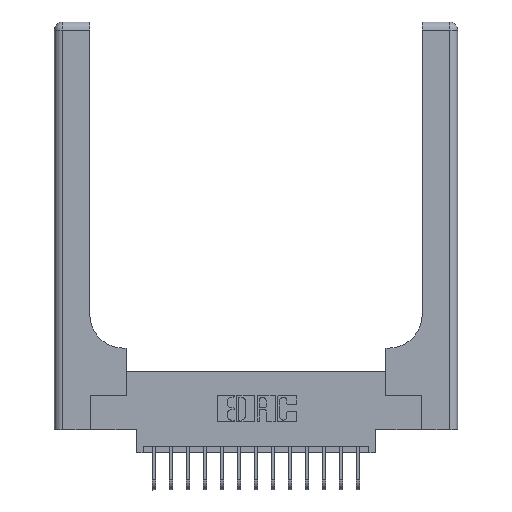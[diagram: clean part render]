
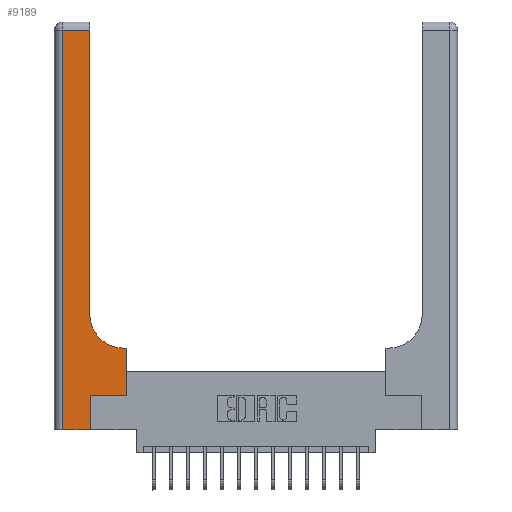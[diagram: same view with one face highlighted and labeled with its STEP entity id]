
A CAD part, top view. The second image highlights one B-rep face of the part: STEP entity #9189.
In plain terms, the highlighted planar face has unit normal (0, 0, 1).
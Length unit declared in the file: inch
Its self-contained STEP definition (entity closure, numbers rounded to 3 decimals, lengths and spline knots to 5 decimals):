
#26 = DIRECTION ( 'NONE',  ( 0., 0., -1. ) ) ;
#106 = CARTESIAN_POINT ( 'NONE',  ( 0.528, 0.25, 0.37 ) ) ;
#921 = VERTEX_POINT ( 'NONE', #11415 ) ;
#1270 = ORIENTED_EDGE ( 'NONE', *, *, #2033, .T. ) ;
#1324 = EDGE_CURVE ( 'NONE', #6707, #921, #7881, .T. ) ;
#1332 = CARTESIAN_POINT ( 'NONE',  ( 0.265, 0.25, 0.37 ) ) ;
#1416 = DIRECTION ( 'NONE',  ( 1., 0., 0. ) ) ;
#1627 = LINE ( 'NONE', #106, #6338 ) ;
#2033 = EDGE_CURVE ( 'NONE', #17599, #7327, #18472, .T. ) ;
#2275 = VERTEX_POINT ( 'NONE', #7486 ) ;
#2289 = EDGE_CURVE ( 'NONE', #13802, #9643, #6070, .T. ) ;
#2573 = VERTEX_POINT ( 'NONE', #11495 ) ;
#2879 = CARTESIAN_POINT ( 'NONE',  ( 0., 3., 0.37 ) ) ;
#3080 = EDGE_CURVE ( 'NONE', #2573, #6707, #17829, .T. ) ;
#3231 = ORIENTED_EDGE ( 'NONE', *, *, #6106, .T. ) ;
#3251 = DIRECTION ( 'NONE',  ( 0., 1., 0. ) ) ;
#3326 = CARTESIAN_POINT ( 'NONE',  ( 0.06, 3., 0.37 ) ) ;
#4124 = CARTESIAN_POINT ( 'NONE',  ( 0.528, 0.25, 0.37 ) ) ;
#4389 = FACE_OUTER_BOUND ( 'NONE', #15207, .T. ) ;
#4398 = EDGE_CURVE ( 'NONE', #5051, #17599, #1627, .T. ) ;
#4751 = DIRECTION ( 'NONE',  ( 0., -1., 0. ) ) ;
#4932 = ORIENTED_EDGE ( 'NONE', *, *, #8261, .T. ) ;
#5051 = VERTEX_POINT ( 'NONE', #4124 ) ;
#5181 = DIRECTION ( 'NONE',  ( 1., 0., 0. ) ) ;
#5896 = ORIENTED_EDGE ( 'NONE', *, *, #12266, .T. ) ;
#6070 = LINE ( 'NONE', #8895, #14020 ) ;
#6106 = EDGE_CURVE ( 'NONE', #7327, #2275, #11852, .T. ) ;
#6338 = VECTOR ( 'NONE', #3251, 39.37008 ) ;
#6693 = CARTESIAN_POINT ( 'NONE',  ( 0.26, 3., 0.37 ) ) ;
#6707 = VERTEX_POINT ( 'NONE', #19014 ) ;
#6904 = DIRECTION ( 'NONE',  ( 0., 1., 0. ) ) ;
#6920 = VECTOR ( 'NONE', #4751, 39.37008 ) ;
#7141 = CARTESIAN_POINT ( 'NONE',  ( 0.26, 0.6, 0.37 ) ) ;
#7327 = VERTEX_POINT ( 'NONE', #10145 ) ;
#7475 = DIRECTION ( 'NONE',  ( 0., 0., -1. ) ) ;
#7486 = CARTESIAN_POINT ( 'NONE',  ( 0.26, 0.85, 0.37 ) ) ;
#7881 = LINE ( 'NONE', #3326, #6920 ) ;
#8017 = EDGE_CURVE ( 'NONE', #921, #13802, #8300, .T. ) ;
#8110 = CARTESIAN_POINT ( 'NONE',  ( 0.528, 0.6, 0.37 ) ) ;
#8261 = EDGE_CURVE ( 'NONE', #9643, #5051, #15157, .T. ) ;
#8300 = LINE ( 'NONE', #18966, #10234 ) ;
#8419 = ORIENTED_EDGE ( 'NONE', *, *, #4398, .T. ) ;
#8660 = VECTOR ( 'NONE', #1416, 39.37008 ) ;
#8895 = CARTESIAN_POINT ( 'NONE',  ( 0.265, 0., 0.37 ) ) ;
#9189 = ADVANCED_FACE ( 'NONE', ( #4389 ), #16714, .F. ) ;
#9643 = VERTEX_POINT ( 'NONE', #15859 ) ;
#10145 = CARTESIAN_POINT ( 'NONE',  ( 0.51, 0.6, 0.37 ) ) ;
#10156 = CARTESIAN_POINT ( 'NONE',  ( 0., 2.94, 0.37 ) ) ;
#10234 = VECTOR ( 'NONE', #5181, 39.37008 ) ;
#10380 = ORIENTED_EDGE ( 'NONE', *, *, #3080, .T. ) ;
#10494 = VECTOR ( 'NONE', #19528, 39.37008 ) ;
#10781 = VECTOR ( 'NONE', #18287, 39.37008 ) ;
#11415 = CARTESIAN_POINT ( 'NONE',  ( 0.06, 0., 0.37 ) ) ;
#11495 = CARTESIAN_POINT ( 'NONE',  ( 0.26, 2.94, 0.37 ) ) ;
#11852 = CIRCLE ( 'NONE', #13165, 0.25 ) ;
#12220 = AXIS2_PLACEMENT_3D ( 'NONE', #2879, #26, #15277 ) ;
#12266 = EDGE_CURVE ( 'NONE', #2275, #2573, #14577, .T. ) ;
#12301 = CARTESIAN_POINT ( 'NONE',  ( 0.51, 0.85, 0.37 ) ) ;
#13165 = AXIS2_PLACEMENT_3D ( 'NONE', #12301, #7475, #17061 ) ;
#13802 = VERTEX_POINT ( 'NONE', #16172 ) ;
#14020 = VECTOR ( 'NONE', #15351, 39.37008 ) ;
#14113 = ORIENTED_EDGE ( 'NONE', *, *, #8017, .T. ) ;
#14577 = LINE ( 'NONE', #6693, #15533 ) ;
#15157 = LINE ( 'NONE', #1332, #8660 ) ;
#15207 = EDGE_LOOP ( 'NONE', ( #5896, #10380, #17522, #14113, #15241, #4932, #8419, #1270, #3231 ) ) ;
#15241 = ORIENTED_EDGE ( 'NONE', *, *, #2289, .T. ) ;
#15277 = DIRECTION ( 'NONE',  ( -1., 0., 0. ) ) ;
#15351 = DIRECTION ( 'NONE',  ( 0., 1., 0. ) ) ;
#15533 = VECTOR ( 'NONE', #6904, 39.37008 ) ;
#15859 = CARTESIAN_POINT ( 'NONE',  ( 0.265, 0.25, 0.37 ) ) ;
#16172 = CARTESIAN_POINT ( 'NONE',  ( 0.265, 0., 0.37 ) ) ;
#16714 = PLANE ( 'NONE',  #12220 ) ;
#17061 = DIRECTION ( 'NONE',  ( 1., 0., 0. ) ) ;
#17522 = ORIENTED_EDGE ( 'NONE', *, *, #1324, .T. ) ;
#17599 = VERTEX_POINT ( 'NONE', #8110 ) ;
#17829 = LINE ( 'NONE', #10156, #10494 ) ;
#18287 = DIRECTION ( 'NONE',  ( -1., 0., 0. ) ) ;
#18472 = LINE ( 'NONE', #7141, #10781 ) ;
#18966 = CARTESIAN_POINT ( 'NONE',  ( 0., 0., 0.37 ) ) ;
#19014 = CARTESIAN_POINT ( 'NONE',  ( 0.06, 2.94, 0.37 ) ) ;
#19528 = DIRECTION ( 'NONE',  ( -1., 0., 0. ) ) ;
